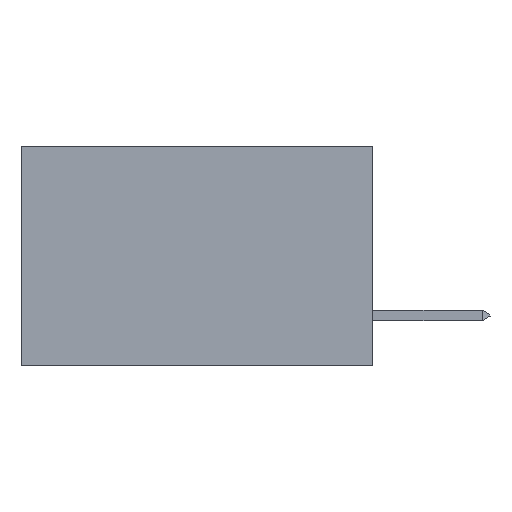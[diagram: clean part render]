
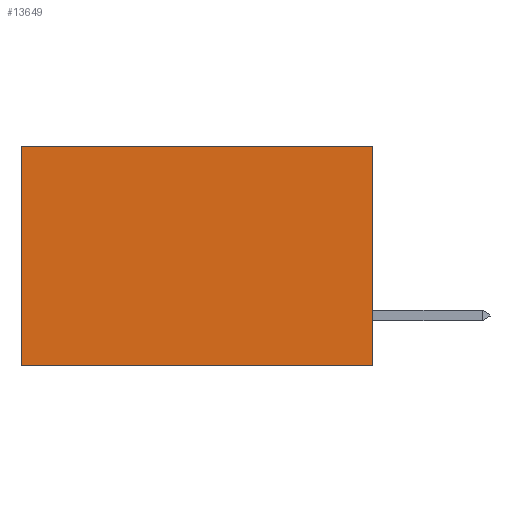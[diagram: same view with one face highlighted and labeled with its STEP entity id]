
A CAD part, left-side view. The second image highlights one B-rep face of the part: STEP entity #13649.
In plain terms, the highlighted planar face has unit normal (-1, 0, 0).
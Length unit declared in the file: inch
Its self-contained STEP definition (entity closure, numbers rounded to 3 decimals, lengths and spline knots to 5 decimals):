
#762 = AXIS2_PLACEMENT_3D ( 'NONE', #19094, #7130, #21101 ) ;
#1060 = CARTESIAN_POINT ( 'NONE',  ( 0.277, 0.59, 0. ) ) ;
#1276 = EDGE_LOOP ( 'NONE', ( #23225, #12767, #19551, #5044 ) ) ;
#1307 = LINE ( 'NONE', #12212, #21984 ) ;
#2744 = VERTEX_POINT ( 'NONE', #11606 ) ;
#3398 = LINE ( 'NONE', #5215, #13444 ) ;
#3892 = VERTEX_POINT ( 'NONE', #10706 ) ;
#5044 = ORIENTED_EDGE ( 'NONE', *, *, #22281, .T. ) ;
#5215 = CARTESIAN_POINT ( 'NONE',  ( 0.277, 0., -0.37 ) ) ;
#7130 = DIRECTION ( 'NONE',  ( 1., 0., 0. ) ) ;
#8245 = DIRECTION ( 'NONE',  ( 0., 1., 0. ) ) ;
#9286 = DIRECTION ( 'NONE',  ( 0., 1., 0. ) ) ;
#10706 = CARTESIAN_POINT ( 'NONE',  ( 0.277, 0., 0. ) ) ;
#10897 = EDGE_CURVE ( 'NONE', #19370, #2744, #21724, .T. ) ;
#11606 = CARTESIAN_POINT ( 'NONE',  ( 0.277, 0.59, -0.37 ) ) ;
#12212 = CARTESIAN_POINT ( 'NONE',  ( 0.277, 0., -0.37 ) ) ;
#12564 = CARTESIAN_POINT ( 'NONE',  ( 0.277, 0., -0.37 ) ) ;
#12767 = ORIENTED_EDGE ( 'NONE', *, *, #23551, .F. ) ;
#13314 = CARTESIAN_POINT ( 'NONE',  ( 0.277, 0., 0. ) ) ;
#13444 = VECTOR ( 'NONE', #21184, 39.37008 ) ;
#13649 = ADVANCED_FACE ( 'NONE', ( #22554 ), #17090, .F. ) ;
#17090 = PLANE ( 'NONE',  #762 ) ;
#18007 = EDGE_CURVE ( 'NONE', #3892, #18468, #3398, .T. ) ;
#18468 = VERTEX_POINT ( 'NONE', #12564 ) ;
#18828 = VECTOR ( 'NONE', #9286, 39.37008 ) ;
#19094 = CARTESIAN_POINT ( 'NONE',  ( 0.277, 0., -0.37 ) ) ;
#19370 = VERTEX_POINT ( 'NONE', #1060 ) ;
#19551 = ORIENTED_EDGE ( 'NONE', *, *, #18007, .F. ) ;
#21101 = DIRECTION ( 'NONE',  ( 0., 0., -1. ) ) ;
#21184 = DIRECTION ( 'NONE',  ( 0., 0., -1. ) ) ;
#21724 = LINE ( 'NONE', #24226, #25706 ) ;
#21984 = VECTOR ( 'NONE', #8245, 39.37008 ) ;
#22281 = EDGE_CURVE ( 'NONE', #3892, #19370, #24098, .T. ) ;
#22353 = DIRECTION ( 'NONE',  ( 0., 0., -1. ) ) ;
#22554 = FACE_OUTER_BOUND ( 'NONE', #1276, .T. ) ;
#23225 = ORIENTED_EDGE ( 'NONE', *, *, #10897, .T. ) ;
#23551 = EDGE_CURVE ( 'NONE', #18468, #2744, #1307, .T. ) ;
#24098 = LINE ( 'NONE', #13314, #18828 ) ;
#24226 = CARTESIAN_POINT ( 'NONE',  ( 0.277, 0.59, -0.37 ) ) ;
#25706 = VECTOR ( 'NONE', #22353, 39.37008 ) ;
